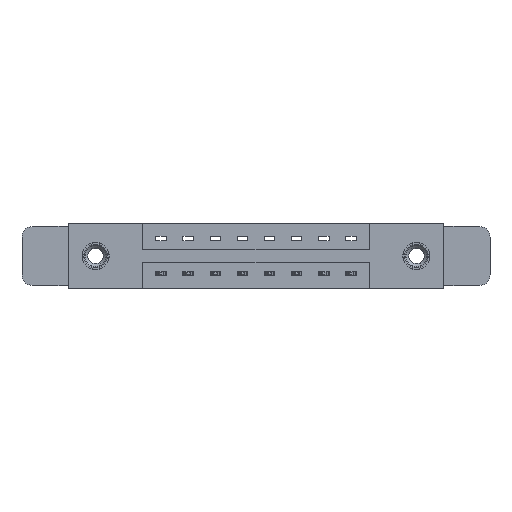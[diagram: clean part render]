
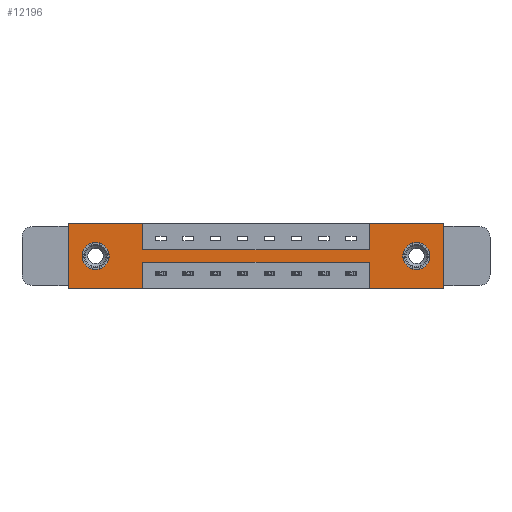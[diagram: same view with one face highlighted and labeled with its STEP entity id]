
A CAD part, front view. The second image highlights one B-rep face of the part: STEP entity #12196.
In plain terms, the highlighted planar face has unit normal (0, -1, 0).
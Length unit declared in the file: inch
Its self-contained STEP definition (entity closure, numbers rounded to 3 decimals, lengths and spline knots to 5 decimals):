
#71 = DIRECTION ( 'NONE',  ( 0., 1., 0. ) ) ;
#89 = CIRCLE ( 'NONE', #4246, 0.078 ) ;
#136 = ORIENTED_EDGE ( 'NONE', *, *, #2915, .T. ) ;
#150 = EDGE_CURVE ( 'NONE', #11949, #1498, #2965, .T. ) ;
#259 = CARTESIAN_POINT ( 'NONE',  ( 2.154, 0., -0.37 ) ) ;
#332 = EDGE_CURVE ( 'NONE', #8915, #1612, #2330, .T. ) ;
#333 = DIRECTION ( 'NONE',  ( -1., 0., 0. ) ) ;
#343 = LINE ( 'NONE', #10387, #10702 ) ;
#460 = CARTESIAN_POINT ( 'NONE',  ( 0., 0., 0. ) ) ;
#692 = ORIENTED_EDGE ( 'NONE', *, *, #6486, .T. ) ;
#731 = FACE_BOUND ( 'NONE', #7909, .T. ) ;
#740 = VECTOR ( 'NONE', #12752, 39.37008 ) ;
#1371 = CARTESIAN_POINT ( 'NONE',  ( 0., 0., -0.37 ) ) ;
#1498 = VERTEX_POINT ( 'NONE', #4393 ) ;
#1598 = VERTEX_POINT ( 'NONE', #10008 ) ;
#1612 = VERTEX_POINT ( 'NONE', #5008 ) ;
#1652 = CIRCLE ( 'NONE', #1683, 0.078 ) ;
#1683 = AXIS2_PLACEMENT_3D ( 'NONE', #8083, #71, #9141 ) ;
#1744 = ORIENTED_EDGE ( 'NONE', *, *, #4711, .F. ) ;
#2203 = VERTEX_POINT ( 'NONE', #8830 ) ;
#2305 = VECTOR ( 'NONE', #4954, 39.37008 ) ;
#2330 = LINE ( 'NONE', #460, #7024 ) ;
#2869 = VERTEX_POINT ( 'NONE', #7154 ) ;
#2871 = VERTEX_POINT ( 'NONE', #10987 ) ;
#2906 = DIRECTION ( 'NONE',  ( 0., 0., -1. ) ) ;
#2915 = EDGE_CURVE ( 'NONE', #4685, #3674, #9955, .T. ) ;
#2965 = LINE ( 'NONE', #10124, #12226 ) ;
#3160 = DIRECTION ( 'NONE',  ( 1., 0., 0. ) ) ;
#3180 = CARTESIAN_POINT ( 'NONE',  ( 0.425, 0., -0.37 ) ) ;
#3276 = EDGE_CURVE ( 'NONE', #8813, #2869, #9692, .T. ) ;
#3281 = ORIENTED_EDGE ( 'NONE', *, *, #6706, .F. ) ;
#3382 = CARTESIAN_POINT ( 'NONE',  ( 0.425, 0., -0.15 ) ) ;
#3489 = CARTESIAN_POINT ( 'NONE',  ( 1.729, 0., 0. ) ) ;
#3512 = EDGE_LOOP ( 'NONE', ( #1744, #4429, #6895, #9167, #3281, #6949, #12951, #11822, #10661, #7011, #7032, #8814 ) ) ;
#3659 = LINE ( 'NONE', #10717, #10570 ) ;
#3674 = VERTEX_POINT ( 'NONE', #12615 ) ;
#3960 = CIRCLE ( 'NONE', #5676, 0.078 ) ;
#3963 = LINE ( 'NONE', #4088, #5852 ) ;
#3986 = VERTEX_POINT ( 'NONE', #9754 ) ;
#4088 = CARTESIAN_POINT ( 'NONE',  ( 2.154, 0., 0. ) ) ;
#4246 = AXIS2_PLACEMENT_3D ( 'NONE', #10883, #8895, #6754 ) ;
#4372 = DIRECTION ( 'NONE',  ( 0., 0., 1. ) ) ;
#4393 = CARTESIAN_POINT ( 'NONE',  ( 1.729, 0., -0.15 ) ) ;
#4429 = ORIENTED_EDGE ( 'NONE', *, *, #12416, .F. ) ;
#4685 = VERTEX_POINT ( 'NONE', #12730 ) ;
#4711 = EDGE_CURVE ( 'NONE', #2203, #12548, #9490, .T. ) ;
#4732 = EDGE_CURVE ( 'NONE', #2871, #1598, #89, .T. ) ;
#4761 = DIRECTION ( 'NONE',  ( 0., 0., -1. ) ) ;
#4907 = PLANE ( 'NONE',  #12244 ) ;
#4910 = VECTOR ( 'NONE', #4761, 39.37008 ) ;
#4934 = CARTESIAN_POINT ( 'NONE',  ( 0.425, 0., 0. ) ) ;
#4954 = DIRECTION ( 'NONE',  ( -1., 0., 0. ) ) ;
#4982 = VECTOR ( 'NONE', #8959, 39.37008 ) ;
#5008 = CARTESIAN_POINT ( 'NONE',  ( 0., 0., 0. ) ) ;
#5256 = DIRECTION ( 'NONE',  ( 0., 1., 0. ) ) ;
#5457 = VERTEX_POINT ( 'NONE', #10515 ) ;
#5671 = CARTESIAN_POINT ( 'NONE',  ( 0.425, 0., -0.22 ) ) ;
#5676 = AXIS2_PLACEMENT_3D ( 'NONE', #6448, #5256, #6406 ) ;
#5679 = EDGE_CURVE ( 'NONE', #5680, #11949, #6634, .T. ) ;
#5680 = VERTEX_POINT ( 'NONE', #7861 ) ;
#5697 = EDGE_CURVE ( 'NONE', #1598, #2871, #1652, .T. ) ;
#5705 = DIRECTION ( 'NONE',  ( 1., 0., 0. ) ) ;
#5720 = CARTESIAN_POINT ( 'NONE',  ( 1.729, 0., 0. ) ) ;
#5808 = EDGE_CURVE ( 'NONE', #1612, #5680, #3659, .T. ) ;
#5852 = VECTOR ( 'NONE', #11116, 39.37008 ) ;
#6059 = LINE ( 'NONE', #12108, #2305 ) ;
#6406 = DIRECTION ( 'NONE',  ( 0., 0., -1. ) ) ;
#6448 = CARTESIAN_POINT ( 'NONE',  ( 1.999, 0., -0.185 ) ) ;
#6486 = EDGE_CURVE ( 'NONE', #3674, #4685, #3960, .T. ) ;
#6634 = LINE ( 'NONE', #4934, #4910 ) ;
#6674 = EDGE_LOOP ( 'NONE', ( #136, #692 ) ) ;
#6706 = EDGE_CURVE ( 'NONE', #3986, #8813, #3963, .T. ) ;
#6754 = DIRECTION ( 'NONE',  ( 0., 0., 1. ) ) ;
#6895 = ORIENTED_EDGE ( 'NONE', *, *, #7587, .F. ) ;
#6923 = CARTESIAN_POINT ( 'NONE',  ( 0., 0., -0.37 ) ) ;
#6949 = ORIENTED_EDGE ( 'NONE', *, *, #9744, .F. ) ;
#7011 = ORIENTED_EDGE ( 'NONE', *, *, #5808, .F. ) ;
#7020 = VECTOR ( 'NONE', #333, 39.37008 ) ;
#7024 = VECTOR ( 'NONE', #10489, 39.37008 ) ;
#7032 = ORIENTED_EDGE ( 'NONE', *, *, #332, .F. ) ;
#7154 = CARTESIAN_POINT ( 'NONE',  ( 1.729, 0., -0.37 ) ) ;
#7266 = FACE_BOUND ( 'NONE', #6674, .T. ) ;
#7269 = VECTOR ( 'NONE', #2906, 39.37008 ) ;
#7587 = EDGE_CURVE ( 'NONE', #2869, #5457, #343, .T. ) ;
#7861 = CARTESIAN_POINT ( 'NONE',  ( 0.425, 0., 0. ) ) ;
#7909 = EDGE_LOOP ( 'NONE', ( #10084, #12783 ) ) ;
#8083 = CARTESIAN_POINT ( 'NONE',  ( 0.155, 0., -0.185 ) ) ;
#8553 = LINE ( 'NONE', #5720, #740 ) ;
#8671 = AXIS2_PLACEMENT_3D ( 'NONE', #12488, #9324, #11392 ) ;
#8764 = CARTESIAN_POINT ( 'NONE',  ( 0.425, 0., -0.37 ) ) ;
#8808 = DIRECTION ( 'NONE',  ( 0., -1., 0. ) ) ;
#8813 = VERTEX_POINT ( 'NONE', #259 ) ;
#8814 = ORIENTED_EDGE ( 'NONE', *, *, #10435, .F. ) ;
#8830 = CARTESIAN_POINT ( 'NONE',  ( 0.425, 0., -0.22 ) ) ;
#8895 = DIRECTION ( 'NONE',  ( 0., 1., 0. ) ) ;
#8915 = VERTEX_POINT ( 'NONE', #9540 ) ;
#8943 = DIRECTION ( 'NONE',  ( 0., 0., -1. ) ) ;
#8959 = DIRECTION ( 'NONE',  ( 1., 0., 0. ) ) ;
#9141 = DIRECTION ( 'NONE',  ( 0., 0., 1. ) ) ;
#9167 = ORIENTED_EDGE ( 'NONE', *, *, #3276, .F. ) ;
#9324 = DIRECTION ( 'NONE',  ( 0., 1., 0. ) ) ;
#9490 = LINE ( 'NONE', #8764, #7269 ) ;
#9540 = CARTESIAN_POINT ( 'NONE',  ( 0., 0., -0.37 ) ) ;
#9692 = LINE ( 'NONE', #1371, #7020 ) ;
#9744 = EDGE_CURVE ( 'NONE', #11171, #3986, #12847, .T. ) ;
#9754 = CARTESIAN_POINT ( 'NONE',  ( 2.154, 0., 0. ) ) ;
#9955 = CIRCLE ( 'NONE', #8671, 0.078 ) ;
#10008 = CARTESIAN_POINT ( 'NONE',  ( 0.155, 0., -0.263 ) ) ;
#10084 = ORIENTED_EDGE ( 'NONE', *, *, #4732, .T. ) ;
#10124 = CARTESIAN_POINT ( 'NONE',  ( 0.425, 0., -0.15 ) ) ;
#10387 = CARTESIAN_POINT ( 'NONE',  ( 1.729, 0., -0.37 ) ) ;
#10435 = EDGE_CURVE ( 'NONE', #12548, #8915, #6059, .T. ) ;
#10489 = DIRECTION ( 'NONE',  ( 0., 0., 1. ) ) ;
#10515 = CARTESIAN_POINT ( 'NONE',  ( 1.729, 0., -0.22 ) ) ;
#10570 = VECTOR ( 'NONE', #5705, 39.37008 ) ;
#10661 = ORIENTED_EDGE ( 'NONE', *, *, #5679, .F. ) ;
#10702 = VECTOR ( 'NONE', #4372, 39.37008 ) ;
#10717 = CARTESIAN_POINT ( 'NONE',  ( 0., 0., 0. ) ) ;
#10883 = CARTESIAN_POINT ( 'NONE',  ( 0.155, 0., -0.185 ) ) ;
#10987 = CARTESIAN_POINT ( 'NONE',  ( 0.155, 0., -0.107 ) ) ;
#11032 = CARTESIAN_POINT ( 'NONE',  ( 0., 0., 0. ) ) ;
#11070 = VECTOR ( 'NONE', #11710, 39.37008 ) ;
#11116 = DIRECTION ( 'NONE',  ( 0., 0., -1. ) ) ;
#11171 = VERTEX_POINT ( 'NONE', #3489 ) ;
#11392 = DIRECTION ( 'NONE',  ( 0., 0., -1. ) ) ;
#11395 = EDGE_CURVE ( 'NONE', #1498, #11171, #8553, .T. ) ;
#11528 = FACE_OUTER_BOUND ( 'NONE', #3512, .T. ) ;
#11694 = LINE ( 'NONE', #5671, #11070 ) ;
#11710 = DIRECTION ( 'NONE',  ( -1., 0., 0. ) ) ;
#11822 = ORIENTED_EDGE ( 'NONE', *, *, #150, .F. ) ;
#11949 = VERTEX_POINT ( 'NONE', #3382 ) ;
#12108 = CARTESIAN_POINT ( 'NONE',  ( 0., 0., -0.37 ) ) ;
#12196 = ADVANCED_FACE ( 'NONE', ( #7266, #731, #11528 ), #4907, .T. ) ;
#12226 = VECTOR ( 'NONE', #3160, 39.37008 ) ;
#12244 = AXIS2_PLACEMENT_3D ( 'NONE', #6923, #8808, #8943 ) ;
#12416 = EDGE_CURVE ( 'NONE', #5457, #2203, #11694, .T. ) ;
#12488 = CARTESIAN_POINT ( 'NONE',  ( 1.999, 0., -0.185 ) ) ;
#12548 = VERTEX_POINT ( 'NONE', #3180 ) ;
#12615 = CARTESIAN_POINT ( 'NONE',  ( 1.999, 0., -0.263 ) ) ;
#12730 = CARTESIAN_POINT ( 'NONE',  ( 1.999, 0., -0.107 ) ) ;
#12752 = DIRECTION ( 'NONE',  ( 0., 0., 1. ) ) ;
#12783 = ORIENTED_EDGE ( 'NONE', *, *, #5697, .T. ) ;
#12847 = LINE ( 'NONE', #11032, #4982 ) ;
#12951 = ORIENTED_EDGE ( 'NONE', *, *, #11395, .F. ) ;
